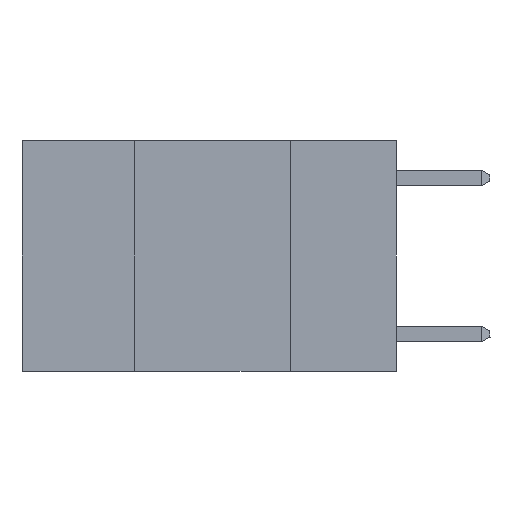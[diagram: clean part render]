
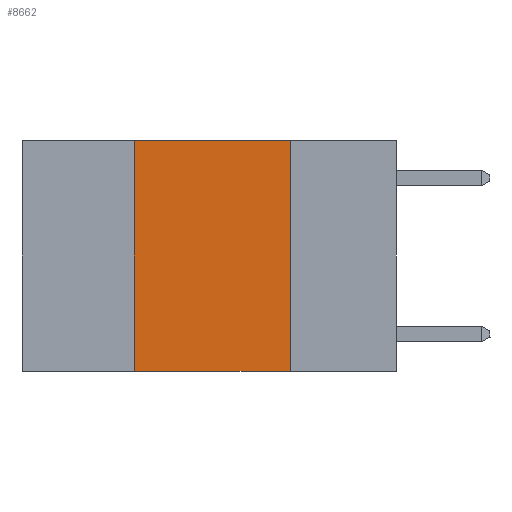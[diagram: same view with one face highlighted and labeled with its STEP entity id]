
A CAD part, left-side view. The second image highlights one B-rep face of the part: STEP entity #8662.
In plain terms, the highlighted planar face has unit normal (-1, 0, 0).
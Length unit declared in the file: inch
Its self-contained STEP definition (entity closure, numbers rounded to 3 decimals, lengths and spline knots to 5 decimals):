
#44 = VERTEX_POINT ( 'NONE', #7908 ) ;
#355 = DIRECTION ( 'NONE',  ( 0., 0., -1. ) ) ;
#679 = VECTOR ( 'NONE', #9791, 39.37008 ) ;
#765 = EDGE_CURVE ( 'NONE', #7483, #12730, #988, .T. ) ;
#988 = LINE ( 'NONE', #8301, #11011 ) ;
#2068 = LINE ( 'NONE', #4096, #7100 ) ;
#2195 = ORIENTED_EDGE ( 'NONE', *, *, #9034, .F. ) ;
#4096 = CARTESIAN_POINT ( 'NONE',  ( 0., 0.17, 0. ) ) ;
#4567 = VERTEX_POINT ( 'NONE', #5514 ) ;
#4800 = LINE ( 'NONE', #10712, #9399 ) ;
#5208 = ORIENTED_EDGE ( 'NONE', *, *, #765, .T. ) ;
#5504 = EDGE_CURVE ( 'NONE', #7483, #4567, #5891, .T. ) ;
#5514 = CARTESIAN_POINT ( 'NONE',  ( 0., 0.42, 0. ) ) ;
#5583 = CARTESIAN_POINT ( 'NONE',  ( 0., 0.6, 0. ) ) ;
#5872 = DIRECTION ( 'NONE',  ( 0., -1., 0. ) ) ;
#5891 = LINE ( 'NONE', #7794, #679 ) ;
#6558 = DIRECTION ( 'NONE',  ( 1., 0., 0. ) ) ;
#6628 = AXIS2_PLACEMENT_3D ( 'NONE', #5583, #6558, #355 ) ;
#7100 = VECTOR ( 'NONE', #9043, 39.37008 ) ;
#7483 = VERTEX_POINT ( 'NONE', #9712 ) ;
#7794 = CARTESIAN_POINT ( 'NONE',  ( 0., 0.42, 0. ) ) ;
#7908 = CARTESIAN_POINT ( 'NONE',  ( 0., 0.17, 0. ) ) ;
#8301 = CARTESIAN_POINT ( 'NONE',  ( 0., 0.6, -0.37 ) ) ;
#8333 = DIRECTION ( 'NONE',  ( 0., -1., 0. ) ) ;
#8498 = FACE_OUTER_BOUND ( 'NONE', #11247, .T. ) ;
#8662 = ADVANCED_FACE ( 'NONE', ( #8498 ), #11391, .F. ) ;
#9034 = EDGE_CURVE ( 'NONE', #44, #12730, #2068, .T. ) ;
#9043 = DIRECTION ( 'NONE',  ( 0., 0., -1. ) ) ;
#9399 = VECTOR ( 'NONE', #5872, 39.37008 ) ;
#9598 = EDGE_CURVE ( 'NONE', #4567, #44, #4800, .T. ) ;
#9712 = CARTESIAN_POINT ( 'NONE',  ( 0., 0.42, -0.37 ) ) ;
#9791 = DIRECTION ( 'NONE',  ( 0., 0., 1. ) ) ;
#10107 = ORIENTED_EDGE ( 'NONE', *, *, #9598, .F. ) ;
#10712 = CARTESIAN_POINT ( 'NONE',  ( 0., 0.6, 0. ) ) ;
#11011 = VECTOR ( 'NONE', #8333, 39.37008 ) ;
#11247 = EDGE_LOOP ( 'NONE', ( #2195, #10107, #12618, #5208 ) ) ;
#11391 = PLANE ( 'NONE',  #6628 ) ;
#12618 = ORIENTED_EDGE ( 'NONE', *, *, #5504, .F. ) ;
#12730 = VERTEX_POINT ( 'NONE', #12771 ) ;
#12771 = CARTESIAN_POINT ( 'NONE',  ( 0., 0.17, -0.37 ) ) ;
